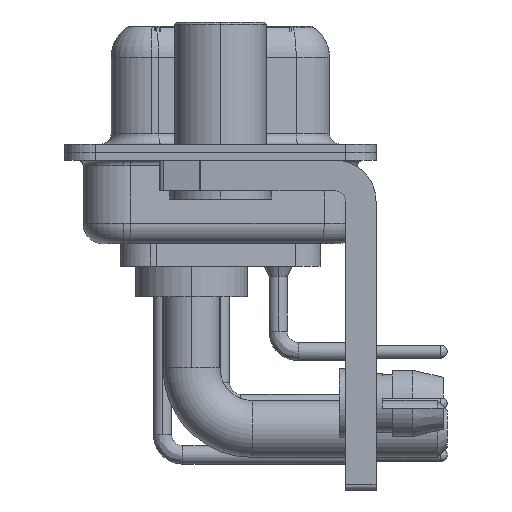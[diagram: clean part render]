
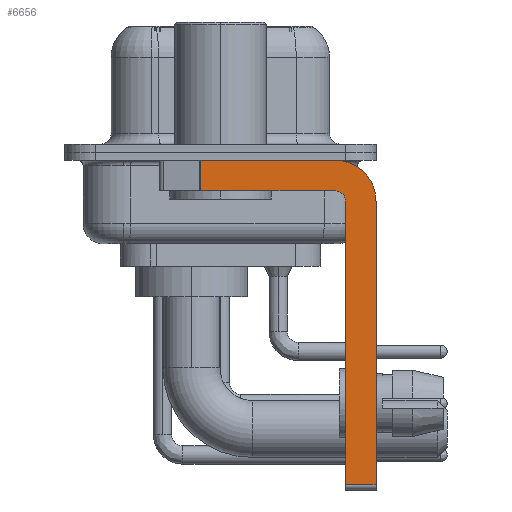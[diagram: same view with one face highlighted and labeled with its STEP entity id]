
A CAD part, left-side view. The second image highlights one B-rep face of the part: STEP entity #6656.
In plain terms, the highlighted planar face has unit normal (-1, 0, 0).
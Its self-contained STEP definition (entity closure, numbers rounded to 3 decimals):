
#259 = CARTESIAN_POINT ( 'NONE',  ( -2.9, -6.15, -16.6 ) ) ;
#1100 = VECTOR ( 'NONE', #15845, 1000. ) ;
#1217 = DIRECTION ( 'NONE',  ( 0., -1., 0. ) ) ;
#1222 = DIRECTION ( 'NONE',  ( 0., -1., 0. ) ) ;
#2338 = EDGE_CURVE ( 'NONE', #9030, #18264, #15165, .T. ) ;
#2881 = EDGE_CURVE ( 'NONE', #14846, #9030, #14628, .T. ) ;
#3215 = DIRECTION ( 'NONE',  ( 1., 0., 0. ) ) ;
#3870 = CARTESIAN_POINT ( 'NONE',  ( -2.9, -5.65, -2.4 ) ) ;
#6123 = CARTESIAN_POINT ( 'NONE',  ( -2.9, -5.65, -2.4 ) ) ;
#6637 = CARTESIAN_POINT ( 'NONE',  ( -2.9, -6.15, -16.35 ) ) ;
#6656 = ADVANCED_FACE ( 'NONE', ( #23414 ), #21034, .F. ) ;
#8177 = CARTESIAN_POINT ( 'NONE',  ( -2.9, 0.978, -0.4 ) ) ;
#8488 = CARTESIAN_POINT ( 'NONE',  ( -2.9, -5.65, -2.4 ) ) ;
#8806 = DIRECTION ( 'NONE',  ( 0., 0., -1. ) ) ;
#9030 = VERTEX_POINT ( 'NONE', #25264 ) ;
#9411 = VERTEX_POINT ( 'NONE', #33015 ) ;
#9532 = LINE ( 'NONE', #29873, #12062 ) ;
#10309 = ORIENTED_EDGE ( 'NONE', *, *, #2338, .F. ) ;
#10340 = DIRECTION ( 'NONE',  ( 0., 0., -1. ) ) ;
#12012 = VECTOR ( 'NONE', #1222, 1000. ) ;
#12030 = CARTESIAN_POINT ( 'NONE',  ( -2.9, -5.65, -16.35 ) ) ;
#12062 = VECTOR ( 'NONE', #32584, 1000. ) ;
#14628 = CIRCLE ( 'NONE', #15729, 0.5 ) ;
#14824 = EDGE_CURVE ( 'NONE', #9411, #22606, #26317, .T. ) ;
#14846 = VERTEX_POINT ( 'NONE', #16751 ) ;
#15085 = CARTESIAN_POINT ( 'NONE',  ( -2.9, -7.65, -16.35 ) ) ;
#15165 = LINE ( 'NONE', #25511, #1100 ) ;
#15729 = AXIS2_PLACEMENT_3D ( 'NONE', #6123, #26312, #31553 ) ;
#15845 = DIRECTION ( 'NONE',  ( 0., 1., 0. ) ) ;
#15938 = CARTESIAN_POINT ( 'NONE',  ( -2.9, -7.65, -2.4 ) ) ;
#16249 = ORIENTED_EDGE ( 'NONE', *, *, #22052, .F. ) ;
#16588 = AXIS2_PLACEMENT_3D ( 'NONE', #3870, #3215, #21852 ) ;
#16609 = LINE ( 'NONE', #15938, #29999 ) ;
#16751 = CARTESIAN_POINT ( 'NONE',  ( -2.9, -6.15, -2.4 ) ) ;
#16772 = EDGE_LOOP ( 'NONE', ( #16249, #21047, #10309, #25752, #22681, #32826, #23051, #23696 ) ) ;
#16879 = CARTESIAN_POINT ( 'NONE',  ( -2.9, 0.978, -1.9 ) ) ;
#17522 = VERTEX_POINT ( 'NONE', #6637 ) ;
#18214 = LINE ( 'NONE', #259, #20623 ) ;
#18264 = VERTEX_POINT ( 'NONE', #16879 ) ;
#20623 = VECTOR ( 'NONE', #26182, 1000. ) ;
#21034 = PLANE ( 'NONE',  #31004 ) ;
#21047 = ORIENTED_EDGE ( 'NONE', *, *, #21629, .T. ) ;
#21629 = EDGE_CURVE ( 'NONE', #28933, #18264, #9532, .T. ) ;
#21852 = DIRECTION ( 'NONE',  ( 0., 0., -1. ) ) ;
#21906 = CARTESIAN_POINT ( 'NONE',  ( -2.9, 3., -0.4 ) ) ;
#22052 = EDGE_CURVE ( 'NONE', #28933, #9411, #27465, .T. ) ;
#22606 = VERTEX_POINT ( 'NONE', #24400 ) ;
#22681 = ORIENTED_EDGE ( 'NONE', *, *, #30908, .F. ) ;
#23051 = ORIENTED_EDGE ( 'NONE', *, *, #23766, .F. ) ;
#23256 = DIRECTION ( 'NONE',  ( 1., 0., 0. ) ) ;
#23414 = FACE_OUTER_BOUND ( 'NONE', #16772, .T. ) ;
#23526 = VERTEX_POINT ( 'NONE', #15085 ) ;
#23696 = ORIENTED_EDGE ( 'NONE', *, *, #14824, .F. ) ;
#23766 = EDGE_CURVE ( 'NONE', #22606, #23526, #16609, .T. ) ;
#24400 = CARTESIAN_POINT ( 'NONE',  ( -2.9, -7.65, -2.4 ) ) ;
#25264 = CARTESIAN_POINT ( 'NONE',  ( -2.9, -5.65, -1.9 ) ) ;
#25511 = CARTESIAN_POINT ( 'NONE',  ( -2.9, -5.65, -1.9 ) ) ;
#25752 = ORIENTED_EDGE ( 'NONE', *, *, #2881, .F. ) ;
#26182 = DIRECTION ( 'NONE',  ( 0., 0., 1. ) ) ;
#26312 = DIRECTION ( 'NONE',  ( -1., 0., 0. ) ) ;
#26317 = CIRCLE ( 'NONE', #16588, 2. ) ;
#27465 = LINE ( 'NONE', #21906, #27827 ) ;
#27470 = LINE ( 'NONE', #12030, #12012 ) ;
#27827 = VECTOR ( 'NONE', #1217, 1000. ) ;
#28933 = VERTEX_POINT ( 'NONE', #8177 ) ;
#29873 = CARTESIAN_POINT ( 'NONE',  ( -2.9, 0.978, -1.9 ) ) ;
#29999 = VECTOR ( 'NONE', #8806, 1000. ) ;
#30908 = EDGE_CURVE ( 'NONE', #17522, #14846, #18214, .T. ) ;
#31004 = AXIS2_PLACEMENT_3D ( 'NONE', #8488, #23256, #10340 ) ;
#31553 = DIRECTION ( 'NONE',  ( 0., 0., 1. ) ) ;
#32584 = DIRECTION ( 'NONE',  ( 0., 0., -1. ) ) ;
#32826 = ORIENTED_EDGE ( 'NONE', *, *, #33360, .T. ) ;
#33015 = CARTESIAN_POINT ( 'NONE',  ( -2.9, -5.65, -0.4 ) ) ;
#33360 = EDGE_CURVE ( 'NONE', #17522, #23526, #27470, .T. ) ;
